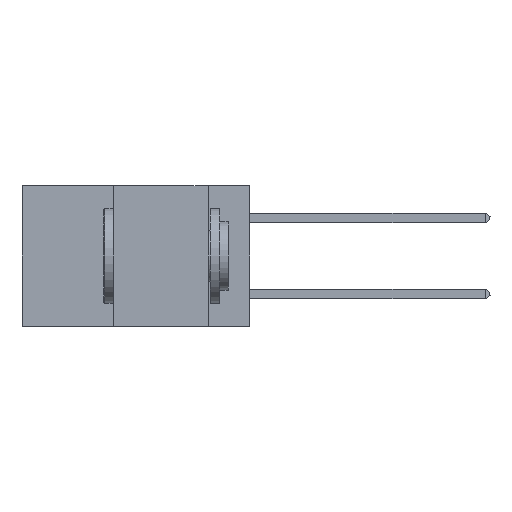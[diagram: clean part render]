
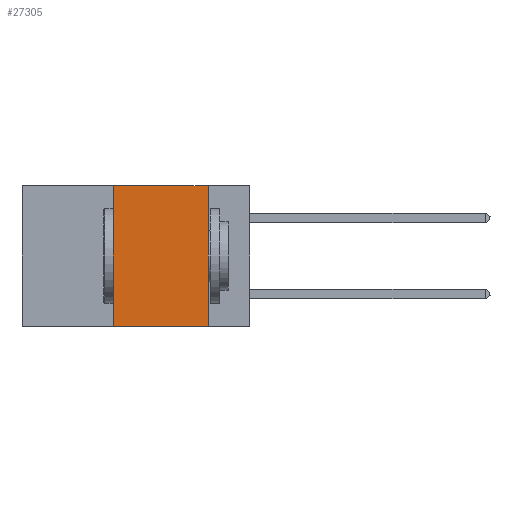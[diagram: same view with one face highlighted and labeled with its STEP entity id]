
A CAD part, left-side view. The second image highlights one B-rep face of the part: STEP entity #27305.
In plain terms, the highlighted planar face has unit normal (-1, 0, 0).
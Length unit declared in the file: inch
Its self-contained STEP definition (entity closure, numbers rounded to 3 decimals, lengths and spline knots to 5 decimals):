
#662 = CARTESIAN_POINT ( 'NONE',  ( 0., 0.36, 0. ) ) ;
#1033 = CARTESIAN_POINT ( 'NONE',  ( 0., 0.6, 0. ) ) ;
#1114 = DIRECTION ( 'NONE',  ( 0., 0., -1. ) ) ;
#1172 = DIRECTION ( 'NONE',  ( 0., 0., -1. ) ) ;
#1696 = LINE ( 'NONE', #20155, #8940 ) ;
#1893 = CARTESIAN_POINT ( 'NONE',  ( 0., 0.36, -0.37 ) ) ;
#2532 = LINE ( 'NONE', #5281, #32653 ) ;
#3457 = FACE_OUTER_BOUND ( 'NONE', #6931, .T. ) ;
#4595 = ORIENTED_EDGE ( 'NONE', *, *, #25826, .F. ) ;
#4993 = VECTOR ( 'NONE', #1114, 39.37008 ) ;
#5281 = CARTESIAN_POINT ( 'NONE',  ( 0., 0.6, 0. ) ) ;
#6931 = EDGE_LOOP ( 'NONE', ( #29499, #10274, #4595, #15548 ) ) ;
#7115 = LINE ( 'NONE', #11775, #15419 ) ;
#8918 = VERTEX_POINT ( 'NONE', #9523 ) ;
#8940 = VECTOR ( 'NONE', #28133, 39.37008 ) ;
#9523 = CARTESIAN_POINT ( 'NONE',  ( 0., 0.11, -0.37 ) ) ;
#10274 = ORIENTED_EDGE ( 'NONE', *, *, #35542, .F. ) ;
#11609 = LINE ( 'NONE', #34120, #4993 ) ;
#11775 = CARTESIAN_POINT ( 'NONE',  ( 0., 0.6, -0.37 ) ) ;
#14568 = DIRECTION ( 'NONE',  ( 0., -1., 0. ) ) ;
#15419 = VECTOR ( 'NONE', #14568, 39.37008 ) ;
#15548 = ORIENTED_EDGE ( 'NONE', *, *, #19356, .T. ) ;
#17285 = EDGE_CURVE ( 'NONE', #34587, #8918, #11609, .T. ) ;
#18093 = DIRECTION ( 'NONE',  ( 1., 0., 0. ) ) ;
#19356 = EDGE_CURVE ( 'NONE', #33501, #8918, #7115, .T. ) ;
#20155 = CARTESIAN_POINT ( 'NONE',  ( 0., 0.36, 0. ) ) ;
#24622 = DIRECTION ( 'NONE',  ( 0., -1., 0. ) ) ;
#25826 = EDGE_CURVE ( 'NONE', #33501, #26434, #1696, .T. ) ;
#26434 = VERTEX_POINT ( 'NONE', #662 ) ;
#27305 = ADVANCED_FACE ( 'NONE', ( #3457 ), #34173, .F. ) ;
#28133 = DIRECTION ( 'NONE',  ( 0., 0., 1. ) ) ;
#29499 = ORIENTED_EDGE ( 'NONE', *, *, #17285, .F. ) ;
#32653 = VECTOR ( 'NONE', #24622, 39.37008 ) ;
#33088 = AXIS2_PLACEMENT_3D ( 'NONE', #1033, #18093, #1172 ) ;
#33501 = VERTEX_POINT ( 'NONE', #1893 ) ;
#34120 = CARTESIAN_POINT ( 'NONE',  ( 0., 0.11, 0. ) ) ;
#34173 = PLANE ( 'NONE',  #33088 ) ;
#34587 = VERTEX_POINT ( 'NONE', #34879 ) ;
#34879 = CARTESIAN_POINT ( 'NONE',  ( 0., 0.11, 0. ) ) ;
#35542 = EDGE_CURVE ( 'NONE', #26434, #34587, #2532, .T. ) ;
